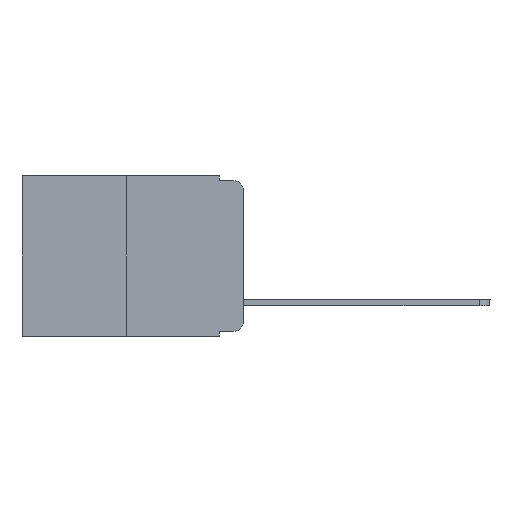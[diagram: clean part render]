
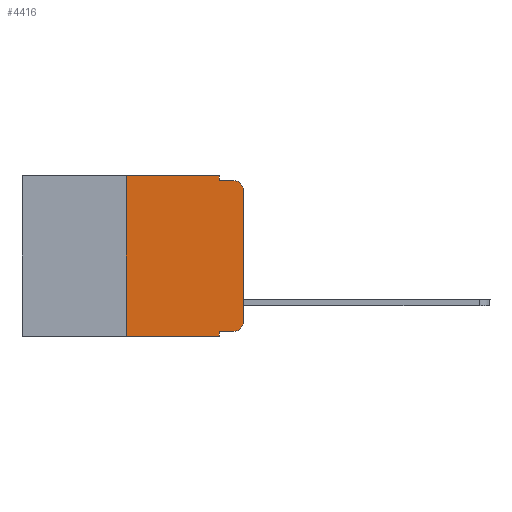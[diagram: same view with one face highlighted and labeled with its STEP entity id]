
A CAD part, left-side view. The second image highlights one B-rep face of the part: STEP entity #4416.
In plain terms, the highlighted planar face has unit normal (-1, 0, 0).
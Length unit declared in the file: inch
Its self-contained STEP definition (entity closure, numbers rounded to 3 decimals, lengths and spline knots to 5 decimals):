
#162 = CARTESIAN_POINT ( 'NONE',  ( 0., 0., 0. ) ) ;
#272 = DIRECTION ( 'NONE',  ( 0., 0., -1. ) ) ;
#636 = DIRECTION ( 'NONE',  ( 0., 0., -1. ) ) ;
#758 = CARTESIAN_POINT ( 'NONE',  ( 0., 0., -0.313 ) ) ;
#1449 = VECTOR ( 'NONE', #272, 39.37008 ) ;
#1632 = VERTEX_POINT ( 'NONE', #15804 ) ;
#1657 = CARTESIAN_POINT ( 'NONE',  ( 0., 0.02, -0.313 ) ) ;
#1702 = VECTOR ( 'NONE', #5474, 39.37008 ) ;
#1836 = ORIENTED_EDGE ( 'NONE', *, *, #12615, .F. ) ;
#2220 = CARTESIAN_POINT ( 'NONE',  ( 0., 0.051, -0.01 ) ) ;
#2227 = ORIENTED_EDGE ( 'NONE', *, *, #16220, .T. ) ;
#2440 = CARTESIAN_POINT ( 'NONE',  ( 0., 0.051, -0.333 ) ) ;
#2535 = LINE ( 'NONE', #15797, #11243 ) ;
#2650 = DIRECTION ( 'NONE',  ( 0., -1., 0. ) ) ;
#2839 = EDGE_CURVE ( 'NONE', #16985, #16487, #11042, .T. ) ;
#3114 = VERTEX_POINT ( 'NONE', #13989 ) ;
#4416 = ADVANCED_FACE ( 'NONE', ( #13641 ), #11110, .F. ) ;
#4480 = CIRCLE ( 'NONE', #15994, 0.02 ) ;
#4490 = AXIS2_PLACEMENT_3D ( 'NONE', #1657, #6983, #16392 ) ;
#4601 = DIRECTION ( 'NONE',  ( 0., -1., 0. ) ) ;
#4876 = EDGE_CURVE ( 'NONE', #5910, #14690, #12552, .T. ) ;
#5162 = EDGE_CURVE ( 'NONE', #11794, #1632, #11772, .T. ) ;
#5368 = VECTOR ( 'NONE', #9691, 39.37008 ) ;
#5376 = ORIENTED_EDGE ( 'NONE', *, *, #5445, .F. ) ;
#5445 = EDGE_CURVE ( 'NONE', #13817, #3114, #6161, .T. ) ;
#5474 = DIRECTION ( 'NONE',  ( 0., 0., 1. ) ) ;
#5874 = EDGE_CURVE ( 'NONE', #14690, #13817, #11018, .T. ) ;
#5910 = VERTEX_POINT ( 'NONE', #8610 ) ;
#6161 = LINE ( 'NONE', #2220, #15162 ) ;
#6324 = VECTOR ( 'NONE', #8394, 39.37008 ) ;
#6376 = ORIENTED_EDGE ( 'NONE', *, *, #12041, .T. ) ;
#6810 = ORIENTED_EDGE ( 'NONE', *, *, #5874, .F. ) ;
#6983 = DIRECTION ( 'NONE',  ( -1., 0., 0. ) ) ;
#7232 = CARTESIAN_POINT ( 'NONE',  ( 0., 0.473, 0. ) ) ;
#7277 = CARTESIAN_POINT ( 'NONE',  ( 0., 0.02, -0.333 ) ) ;
#7319 = ORIENTED_EDGE ( 'NONE', *, *, #15286, .F. ) ;
#7397 = CARTESIAN_POINT ( 'NONE',  ( 0., 0.25, -0.343 ) ) ;
#7566 = DIRECTION ( 'NONE',  ( 0., -1., 0. ) ) ;
#7730 = ORIENTED_EDGE ( 'NONE', *, *, #5162, .T. ) ;
#8376 = CARTESIAN_POINT ( 'NONE',  ( 0., 0.473, 0. ) ) ;
#8394 = DIRECTION ( 'NONE',  ( 0., -1., 0. ) ) ;
#8610 = CARTESIAN_POINT ( 'NONE',  ( 0., 0.25, 0. ) ) ;
#9357 = DIRECTION ( 'NONE',  ( -1., 0., 0. ) ) ;
#9501 = VECTOR ( 'NONE', #4601, 39.37008 ) ;
#9691 = DIRECTION ( 'NONE',  ( 0., 0., -1. ) ) ;
#10533 = ORIENTED_EDGE ( 'NONE', *, *, #13896, .T. ) ;
#10535 = LINE ( 'NONE', #15652, #14650 ) ;
#11018 = LINE ( 'NONE', #16210, #5368 ) ;
#11042 = LINE ( 'NONE', #16412, #6324 ) ;
#11110 = PLANE ( 'NONE',  #13674 ) ;
#11182 = CARTESIAN_POINT ( 'NONE',  ( 0., 0.051, 0. ) ) ;
#11243 = VECTOR ( 'NONE', #13210, 39.37008 ) ;
#11305 = VERTEX_POINT ( 'NONE', #7397 ) ;
#11312 = CARTESIAN_POINT ( 'NONE',  ( 0., 0.051, -0.343 ) ) ;
#11772 = LINE ( 'NONE', #162, #1702 ) ;
#11794 = VERTEX_POINT ( 'NONE', #758 ) ;
#11816 = VERTEX_POINT ( 'NONE', #11312 ) ;
#11908 = CARTESIAN_POINT ( 'NONE',  ( 0., 0.02, -0.03 ) ) ;
#12034 = CIRCLE ( 'NONE', #4490, 0.02 ) ;
#12041 = EDGE_CURVE ( 'NONE', #1632, #3114, #4480, .T. ) ;
#12371 = ORIENTED_EDGE ( 'NONE', *, *, #4876, .F. ) ;
#12552 = LINE ( 'NONE', #7232, #9501 ) ;
#12615 = EDGE_CURVE ( 'NONE', #16985, #11816, #16645, .T. ) ;
#13210 = DIRECTION ( 'NONE',  ( 0., 0., 1. ) ) ;
#13641 = FACE_OUTER_BOUND ( 'NONE', #16924, .T. ) ;
#13674 = AXIS2_PLACEMENT_3D ( 'NONE', #8376, #16657, #636 ) ;
#13817 = VERTEX_POINT ( 'NONE', #16300 ) ;
#13896 = EDGE_CURVE ( 'NONE', #16487, #11794, #12034, .T. ) ;
#13989 = CARTESIAN_POINT ( 'NONE',  ( 0., 0.02, -0.01 ) ) ;
#14650 = VECTOR ( 'NONE', #2650, 39.37008 ) ;
#14690 = VERTEX_POINT ( 'NONE', #15572 ) ;
#15155 = ORIENTED_EDGE ( 'NONE', *, *, #2839, .T. ) ;
#15162 = VECTOR ( 'NONE', #7566, 39.37008 ) ;
#15286 = EDGE_CURVE ( 'NONE', #11305, #5910, #2535, .T. ) ;
#15572 = CARTESIAN_POINT ( 'NONE',  ( 0., 0.051, 0. ) ) ;
#15652 = CARTESIAN_POINT ( 'NONE',  ( 0., 0.473, -0.343 ) ) ;
#15797 = CARTESIAN_POINT ( 'NONE',  ( 0., 0.25, 0. ) ) ;
#15804 = CARTESIAN_POINT ( 'NONE',  ( 0., 0., -0.03 ) ) ;
#15994 = AXIS2_PLACEMENT_3D ( 'NONE', #11908, #9357, #17280 ) ;
#16210 = CARTESIAN_POINT ( 'NONE',  ( 0., 0.051, 0. ) ) ;
#16220 = EDGE_CURVE ( 'NONE', #11305, #11816, #10535, .T. ) ;
#16300 = CARTESIAN_POINT ( 'NONE',  ( 0., 0.051, -0.01 ) ) ;
#16392 = DIRECTION ( 'NONE',  ( 0., 0., -1. ) ) ;
#16412 = CARTESIAN_POINT ( 'NONE',  ( 0., 0.051, -0.333 ) ) ;
#16487 = VERTEX_POINT ( 'NONE', #7277 ) ;
#16645 = LINE ( 'NONE', #11182, #1449 ) ;
#16657 = DIRECTION ( 'NONE',  ( 1., 0., 0. ) ) ;
#16924 = EDGE_LOOP ( 'NONE', ( #7730, #6376, #5376, #6810, #12371, #7319, #2227, #1836, #15155, #10533 ) ) ;
#16985 = VERTEX_POINT ( 'NONE', #2440 ) ;
#17280 = DIRECTION ( 'NONE',  ( 0., 0., -1. ) ) ;
